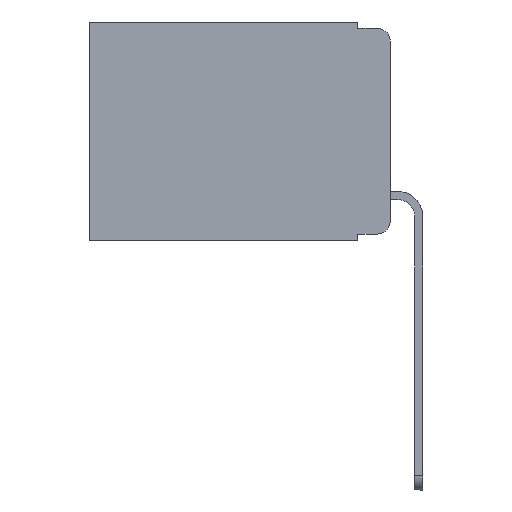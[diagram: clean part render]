
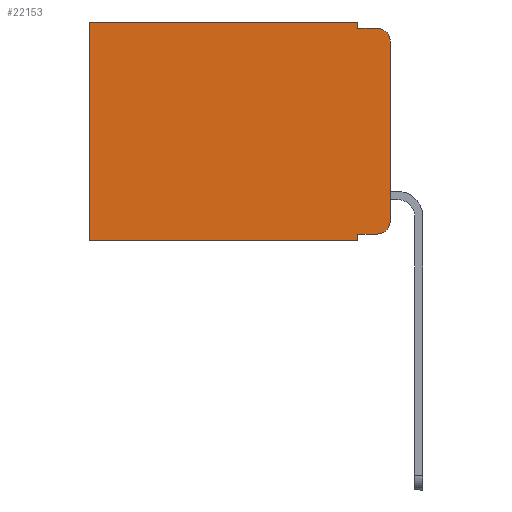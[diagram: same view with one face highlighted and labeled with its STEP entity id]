
A CAD part, left-side view. The second image highlights one B-rep face of the part: STEP entity #22153.
In plain terms, the highlighted planar face has unit normal (-1, 0, 0).
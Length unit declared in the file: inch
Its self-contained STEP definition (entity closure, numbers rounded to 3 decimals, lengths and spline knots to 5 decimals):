
#323 = VERTEX_POINT ( 'NONE', #11882 ) ;
#381 = EDGE_CURVE ( 'NONE', #7932, #8571, #19922, .T. ) ;
#800 = EDGE_CURVE ( 'NONE', #18909, #4051, #4883, .T. ) ;
#1360 = CARTESIAN_POINT ( 'NONE',  ( 0.298, 0.051, 0. ) ) ;
#1515 = EDGE_LOOP ( 'NONE', ( #22774, #3329, #2415, #13400, #18638, #5939, #4650, #17422, #13217, #14883 ) ) ;
#1652 = FACE_OUTER_BOUND ( 'NONE', #1515, .T. ) ;
#1893 = LINE ( 'NONE', #17259, #15328 ) ;
#2015 = LINE ( 'NONE', #6036, #6215 ) ;
#2415 = ORIENTED_EDGE ( 'NONE', *, *, #12529, .F. ) ;
#2719 = DIRECTION ( 'NONE',  ( -1., 0., 0. ) ) ;
#2838 = DIRECTION ( 'NONE',  ( 0., 0., -1. ) ) ;
#2948 = CARTESIAN_POINT ( 'NONE',  ( 0.298, 0.02, -0.01 ) ) ;
#3004 = DIRECTION ( 'NONE',  ( 1., 0., 0. ) ) ;
#3329 = ORIENTED_EDGE ( 'NONE', *, *, #17020, .T. ) ;
#3382 = LINE ( 'NONE', #23981, #13537 ) ;
#4051 = VERTEX_POINT ( 'NONE', #4609 ) ;
#4405 = DIRECTION ( 'NONE',  ( 0., -1., 0. ) ) ;
#4537 = CIRCLE ( 'NONE', #14682, 0.02 ) ;
#4609 = CARTESIAN_POINT ( 'NONE',  ( 0.298, 0.02, -0.333 ) ) ;
#4650 = ORIENTED_EDGE ( 'NONE', *, *, #21487, .F. ) ;
#4883 = LINE ( 'NONE', #6347, #9722 ) ;
#5266 = AXIS2_PLACEMENT_3D ( 'NONE', #12232, #2719, #2838 ) ;
#5477 = EDGE_CURVE ( 'NONE', #8179, #15234, #14132, .T. ) ;
#5565 = DIRECTION ( 'NONE',  ( 0., 0., -1. ) ) ;
#5939 = ORIENTED_EDGE ( 'NONE', *, *, #381, .T. ) ;
#6011 = DIRECTION ( 'NONE',  ( 0., 1., 0. ) ) ;
#6036 = CARTESIAN_POINT ( 'NONE',  ( 0.298, 0., 0. ) ) ;
#6215 = VECTOR ( 'NONE', #22507, 39.37008 ) ;
#6229 = EDGE_CURVE ( 'NONE', #18909, #323, #1893, .T. ) ;
#6347 = CARTESIAN_POINT ( 'NONE',  ( 0.298, 0.051, -0.333 ) ) ;
#6556 = CARTESIAN_POINT ( 'NONE',  ( 0.298, 0., 0. ) ) ;
#7229 = CARTESIAN_POINT ( 'NONE',  ( 0.298, 0., -0.03 ) ) ;
#7847 = CARTESIAN_POINT ( 'NONE',  ( 0.298, 0.473, 0. ) ) ;
#7932 = VERTEX_POINT ( 'NONE', #7847 ) ;
#8179 = VERTEX_POINT ( 'NONE', #1360 ) ;
#8236 = CARTESIAN_POINT ( 'NONE',  ( 0.298, 0.051, -0.01 ) ) ;
#8300 = VERTEX_POINT ( 'NONE', #11105 ) ;
#8571 = VERTEX_POINT ( 'NONE', #8904 ) ;
#8904 = CARTESIAN_POINT ( 'NONE',  ( 0.298, 0.473, -0.343 ) ) ;
#9722 = VECTOR ( 'NONE', #4405, 39.37008 ) ;
#9936 = CIRCLE ( 'NONE', #5266, 0.02 ) ;
#10998 = EDGE_CURVE ( 'NONE', #4051, #8300, #4537, .T. ) ;
#11105 = CARTESIAN_POINT ( 'NONE',  ( 0.298, 0., -0.313 ) ) ;
#11396 = VECTOR ( 'NONE', #23092, 39.37008 ) ;
#11882 = CARTESIAN_POINT ( 'NONE',  ( 0.298, 0.051, -0.343 ) ) ;
#12232 = CARTESIAN_POINT ( 'NONE',  ( 0.298, 0.02, -0.03 ) ) ;
#12529 = EDGE_CURVE ( 'NONE', #15234, #14654, #13579, .T. ) ;
#12836 = DIRECTION ( 'NONE',  ( 0., -1., 0. ) ) ;
#13206 = VECTOR ( 'NONE', #12836, 39.37008 ) ;
#13217 = ORIENTED_EDGE ( 'NONE', *, *, #800, .T. ) ;
#13400 = ORIENTED_EDGE ( 'NONE', *, *, #5477, .F. ) ;
#13537 = VECTOR ( 'NONE', #6011, 39.37008 ) ;
#13579 = LINE ( 'NONE', #14173, #13206 ) ;
#14132 = LINE ( 'NONE', #16328, #23079 ) ;
#14173 = CARTESIAN_POINT ( 'NONE',  ( 0.298, 0.051, -0.01 ) ) ;
#14601 = CARTESIAN_POINT ( 'NONE',  ( 0.298, 0., 0. ) ) ;
#14654 = VERTEX_POINT ( 'NONE', #2948 ) ;
#14682 = AXIS2_PLACEMENT_3D ( 'NONE', #15903, #19319, #21379 ) ;
#14883 = ORIENTED_EDGE ( 'NONE', *, *, #10998, .T. ) ;
#15234 = VERTEX_POINT ( 'NONE', #8236 ) ;
#15328 = VECTOR ( 'NONE', #22856, 39.37008 ) ;
#15903 = CARTESIAN_POINT ( 'NONE',  ( 0.298, 0.02, -0.313 ) ) ;
#15922 = AXIS2_PLACEMENT_3D ( 'NONE', #14601, #3004, #17884 ) ;
#15938 = PLANE ( 'NONE',  #15922 ) ;
#16328 = CARTESIAN_POINT ( 'NONE',  ( 0.298, 0.051, 0. ) ) ;
#17020 = EDGE_CURVE ( 'NONE', #18955, #14654, #9936, .T. ) ;
#17259 = CARTESIAN_POINT ( 'NONE',  ( 0.298, 0.051, 0. ) ) ;
#17422 = ORIENTED_EDGE ( 'NONE', *, *, #6229, .F. ) ;
#17844 = EDGE_CURVE ( 'NONE', #18955, #8300, #19382, .T. ) ;
#17884 = DIRECTION ( 'NONE',  ( 0., 0., -1. ) ) ;
#18137 = VECTOR ( 'NONE', #21320, 39.37008 ) ;
#18638 = ORIENTED_EDGE ( 'NONE', *, *, #23526, .T. ) ;
#18909 = VERTEX_POINT ( 'NONE', #19811 ) ;
#18955 = VERTEX_POINT ( 'NONE', #7229 ) ;
#19319 = DIRECTION ( 'NONE',  ( -1., 0., 0. ) ) ;
#19382 = LINE ( 'NONE', #6556, #18137 ) ;
#19811 = CARTESIAN_POINT ( 'NONE',  ( 0.298, 0.051, -0.333 ) ) ;
#19922 = LINE ( 'NONE', #21262, #11396 ) ;
#21262 = CARTESIAN_POINT ( 'NONE',  ( 0.298, 0.473, 0. ) ) ;
#21320 = DIRECTION ( 'NONE',  ( 0., 0., -1. ) ) ;
#21379 = DIRECTION ( 'NONE',  ( 0., 0., -1. ) ) ;
#21487 = EDGE_CURVE ( 'NONE', #323, #8571, #3382, .T. ) ;
#22153 = ADVANCED_FACE ( 'NONE', ( #1652 ), #15938, .F. ) ;
#22507 = DIRECTION ( 'NONE',  ( 0., 1., 0. ) ) ;
#22774 = ORIENTED_EDGE ( 'NONE', *, *, #17844, .F. ) ;
#22856 = DIRECTION ( 'NONE',  ( 0., 0., -1. ) ) ;
#23079 = VECTOR ( 'NONE', #5565, 39.37008 ) ;
#23092 = DIRECTION ( 'NONE',  ( 0., 0., -1. ) ) ;
#23526 = EDGE_CURVE ( 'NONE', #8179, #7932, #2015, .T. ) ;
#23981 = CARTESIAN_POINT ( 'NONE',  ( 0.298, 0., -0.343 ) ) ;
